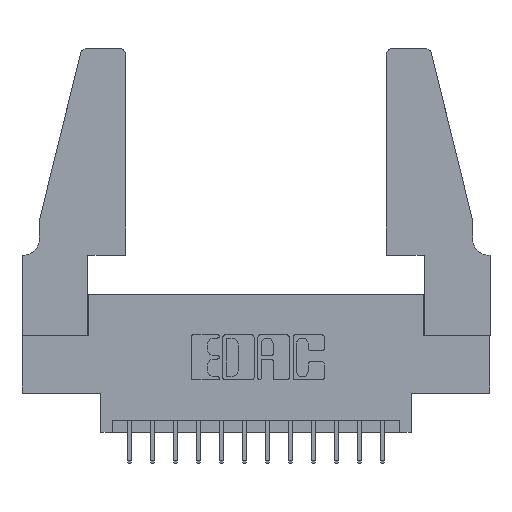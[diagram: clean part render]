
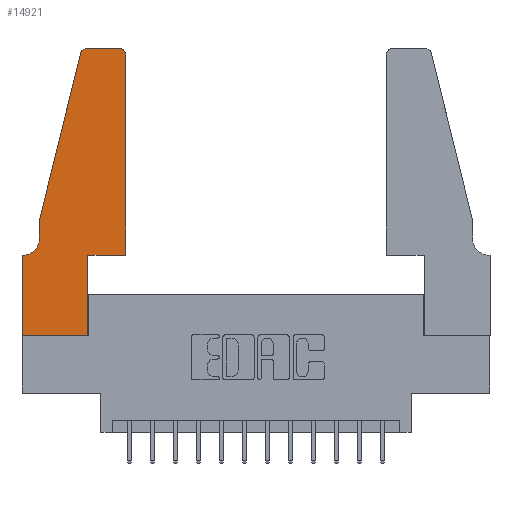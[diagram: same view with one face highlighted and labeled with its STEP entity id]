
A CAD part, top view. The second image highlights one B-rep face of the part: STEP entity #14921.
In plain terms, the highlighted planar face has unit normal (0, 0, 1).
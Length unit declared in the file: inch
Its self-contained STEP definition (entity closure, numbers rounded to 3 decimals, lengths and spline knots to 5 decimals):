
#144 = VERTEX_POINT ( 'NONE', #11113 ) ;
#160 = EDGE_CURVE ( 'NONE', #956, #144, #8530, .T. ) ;
#259 = VECTOR ( 'NONE', #4999, 39.37008 ) ;
#417 = AXIS2_PLACEMENT_3D ( 'NONE', #14358, #5715, #12073 ) ;
#453 = EDGE_CURVE ( 'NONE', #2006, #2160, #15364, .T. ) ;
#515 = VERTEX_POINT ( 'NONE', #9598 ) ;
#636 = VECTOR ( 'NONE', #9134, 39.37008 ) ;
#819 = CARTESIAN_POINT ( 'NONE',  ( 0.4505, 0.35, 0.37 ) ) ;
#916 = FACE_OUTER_BOUND ( 'NONE', #3325, .T. ) ;
#956 = VERTEX_POINT ( 'NONE', #11792 ) ;
#1124 = VECTOR ( 'NONE', #12969, 39.37008 ) ;
#1216 = DIRECTION ( 'NONE',  ( 0., -1., 0. ) ) ;
#1273 = ORIENTED_EDGE ( 'NONE', *, *, #14180, .T. ) ;
#1320 = VERTEX_POINT ( 'NONE', #12551 ) ;
#1835 = CARTESIAN_POINT ( 'NONE',  ( 0.4205, 1.22, 0.37 ) ) ;
#1941 = VERTEX_POINT ( 'NONE', #8501 ) ;
#2006 = VERTEX_POINT ( 'NONE', #13309 ) ;
#2046 = EDGE_CURVE ( 'NONE', #515, #956, #10277, .T. ) ;
#2160 = VERTEX_POINT ( 'NONE', #14893 ) ;
#2423 = AXIS2_PLACEMENT_3D ( 'NONE', #1835, #15366, #5343 ) ;
#2557 = ORIENTED_EDGE ( 'NONE', *, *, #5738, .T. ) ;
#3107 = CARTESIAN_POINT ( 'NONE',  ( 0.4505, 0.35, 0.37 ) ) ;
#3325 = EDGE_LOOP ( 'NONE', ( #4407, #12084, #13163, #6219, #5547, #11572, #1273, #2557, #3382, #10003, #11005, #10808 ) ) ;
#3365 = CARTESIAN_POINT ( 'NONE',  ( 0.2605, 1.25, 0.37 ) ) ;
#3382 = ORIENTED_EDGE ( 'NONE', *, *, #6843, .T. ) ;
#3404 = VERTEX_POINT ( 'NONE', #12566 ) ;
#3639 = DIRECTION ( 'NONE',  ( -1., 0., 0. ) ) ;
#4089 = AXIS2_PLACEMENT_3D ( 'NONE', #14580, #13385, #7276 ) ;
#4407 = ORIENTED_EDGE ( 'NONE', *, *, #11503, .T. ) ;
#4473 = DIRECTION ( 'NONE',  ( 1., 0., 0. ) ) ;
#4851 = VERTEX_POINT ( 'NONE', #819 ) ;
#4917 = CARTESIAN_POINT ( 'NONE',  ( 0., 0., 0.37 ) ) ;
#4999 = DIRECTION ( 'NONE',  ( -0.239, -0.971, 0. ) ) ;
#5343 = DIRECTION ( 'NONE',  ( 1., 0., 0. ) ) ;
#5364 = LINE ( 'NONE', #3107, #12910 ) ;
#5417 = EDGE_CURVE ( 'NONE', #4851, #1941, #7285, .T. ) ;
#5547 = ORIENTED_EDGE ( 'NONE', *, *, #453, .T. ) ;
#5715 = DIRECTION ( 'NONE',  ( 0., 0., 1. ) ) ;
#5738 = EDGE_CURVE ( 'NONE', #7852, #1320, #10515, .T. ) ;
#6219 = ORIENTED_EDGE ( 'NONE', *, *, #10887, .T. ) ;
#6462 = VECTOR ( 'NONE', #14837, 39.37008 ) ;
#6564 = EDGE_CURVE ( 'NONE', #1941, #3404, #8318, .T. ) ;
#6843 = EDGE_CURVE ( 'NONE', #1320, #13704, #13827, .T. ) ;
#6962 = VERTEX_POINT ( 'NONE', #14294 ) ;
#7276 = DIRECTION ( 'NONE',  ( 1., 0., 0. ) ) ;
#7285 = LINE ( 'NONE', #9796, #12126 ) ;
#7360 = VECTOR ( 'NONE', #8290, 39.37008 ) ;
#7457 = DIRECTION ( 'NONE',  ( 0., 1., 0. ) ) ;
#7680 = LINE ( 'NONE', #14810, #12185 ) ;
#7844 = CARTESIAN_POINT ( 'NONE',  ( 0.2865, 0.35, 0.37 ) ) ;
#7852 = VERTEX_POINT ( 'NONE', #4917 ) ;
#8216 = EDGE_CURVE ( 'NONE', #13704, #4851, #5364, .T. ) ;
#8290 = DIRECTION ( 'NONE',  ( -1., 0., 0. ) ) ;
#8318 = CIRCLE ( 'NONE', #2423, 0.03 ) ;
#8436 = LINE ( 'NONE', #14589, #13736 ) ;
#8501 = CARTESIAN_POINT ( 'NONE',  ( 0.4505, 1.22, 0.37 ) ) ;
#8530 = LINE ( 'NONE', #14849, #259 ) ;
#9134 = DIRECTION ( 'NONE',  ( 0., 1., 0. ) ) ;
#9334 = LINE ( 'NONE', #3365, #7360 ) ;
#9598 = CARTESIAN_POINT ( 'NONE',  ( 0.284, 1.25, 0.37 ) ) ;
#9727 = AXIS2_PLACEMENT_3D ( 'NONE', #11126, #14785, #3639 ) ;
#9796 = CARTESIAN_POINT ( 'NONE',  ( 0.4505, 0.35, 0.37 ) ) ;
#9976 = CARTESIAN_POINT ( 'NONE',  ( 0.0755, 0.35, 0.37 ) ) ;
#9996 = EDGE_CURVE ( 'NONE', #2160, #6962, #13401, .T. ) ;
#10003 = ORIENTED_EDGE ( 'NONE', *, *, #8216, .T. ) ;
#10277 = CIRCLE ( 'NONE', #4089, 0.03 ) ;
#10515 = LINE ( 'NONE', #11632, #1124 ) ;
#10574 = CARTESIAN_POINT ( 'NONE',  ( 0.2865, 0.35, 0.37 ) ) ;
#10808 = ORIENTED_EDGE ( 'NONE', *, *, #6564, .T. ) ;
#10887 = EDGE_CURVE ( 'NONE', #144, #2006, #8436, .T. ) ;
#11005 = ORIENTED_EDGE ( 'NONE', *, *, #5417, .T. ) ;
#11073 = DIRECTION ( 'NONE',  ( 0., -1., 0. ) ) ;
#11113 = CARTESIAN_POINT ( 'NONE',  ( 0.0755, 0.5, 0.37 ) ) ;
#11126 = CARTESIAN_POINT ( 'NONE',  ( 0.0055, 0.42, 0.37 ) ) ;
#11503 = EDGE_CURVE ( 'NONE', #3404, #515, #9334, .T. ) ;
#11572 = ORIENTED_EDGE ( 'NONE', *, *, #9996, .T. ) ;
#11632 = CARTESIAN_POINT ( 'NONE',  ( 0., 0., 0.37 ) ) ;
#11792 = CARTESIAN_POINT ( 'NONE',  ( 0.25487, 1.22718, 0.37 ) ) ;
#12073 = DIRECTION ( 'NONE',  ( 1., 0., 0. ) ) ;
#12084 = ORIENTED_EDGE ( 'NONE', *, *, #2046, .T. ) ;
#12126 = VECTOR ( 'NONE', #7457, 39.37008 ) ;
#12185 = VECTOR ( 'NONE', #11073, 39.37008 ) ;
#12551 = CARTESIAN_POINT ( 'NONE',  ( 0.2865, 0., 0.37 ) ) ;
#12566 = CARTESIAN_POINT ( 'NONE',  ( 0.4205, 1.25, 0.37 ) ) ;
#12910 = VECTOR ( 'NONE', #4473, 39.37008 ) ;
#12969 = DIRECTION ( 'NONE',  ( 1., 0., 0. ) ) ;
#13163 = ORIENTED_EDGE ( 'NONE', *, *, #160, .T. ) ;
#13170 = PLANE ( 'NONE',  #417 ) ;
#13309 = CARTESIAN_POINT ( 'NONE',  ( 0.0755, 0.42, 0.37 ) ) ;
#13385 = DIRECTION ( 'NONE',  ( 0., 0., 1. ) ) ;
#13401 = LINE ( 'NONE', #9976, #6462 ) ;
#13704 = VERTEX_POINT ( 'NONE', #10574 ) ;
#13736 = VECTOR ( 'NONE', #1216, 39.37008 ) ;
#13827 = LINE ( 'NONE', #7844, #636 ) ;
#14180 = EDGE_CURVE ( 'NONE', #6962, #7852, #7680, .T. ) ;
#14294 = CARTESIAN_POINT ( 'NONE',  ( 0., 0.35, 0.37 ) ) ;
#14358 = CARTESIAN_POINT ( 'NONE',  ( 0., 0.35, 0.37 ) ) ;
#14580 = CARTESIAN_POINT ( 'NONE',  ( 0.284, 1.22, 0.37 ) ) ;
#14589 = CARTESIAN_POINT ( 'NONE',  ( 0.0755, 0.5, 0.37 ) ) ;
#14785 = DIRECTION ( 'NONE',  ( 0., 0., -1. ) ) ;
#14810 = CARTESIAN_POINT ( 'NONE',  ( 0., 0., 0.37 ) ) ;
#14837 = DIRECTION ( 'NONE',  ( -1., 0., 0. ) ) ;
#14849 = CARTESIAN_POINT ( 'NONE',  ( 0.0755, 0.5, 0.37 ) ) ;
#14893 = CARTESIAN_POINT ( 'NONE',  ( 0.0055, 0.35, 0.37 ) ) ;
#14921 = ADVANCED_FACE ( 'NONE', ( #916 ), #13170, .T. ) ;
#15364 = CIRCLE ( 'NONE', #9727, 0.07 ) ;
#15366 = DIRECTION ( 'NONE',  ( 0., 0., 1. ) ) ;
